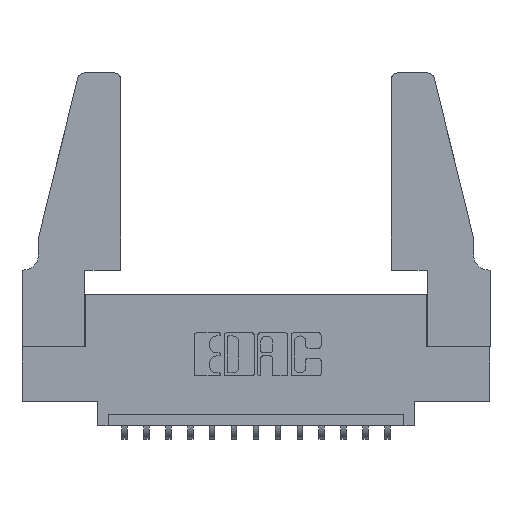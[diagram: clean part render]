
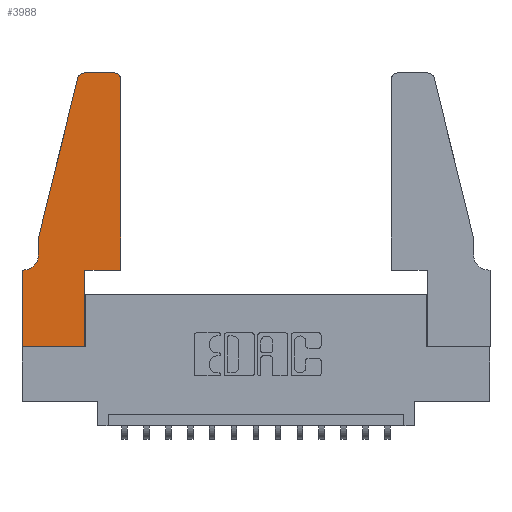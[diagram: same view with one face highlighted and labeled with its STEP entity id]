
A CAD part, top view. The second image highlights one B-rep face of the part: STEP entity #3988.
In plain terms, the highlighted planar face has unit normal (0, 0, 1).
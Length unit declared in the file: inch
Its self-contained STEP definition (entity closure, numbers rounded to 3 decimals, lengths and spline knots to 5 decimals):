
#80 = DIRECTION ( 'NONE',  ( -0.239, -0.971, 0. ) ) ;
#277 = CIRCLE ( 'NONE', #10019, 0.07 ) ;
#354 = ORIENTED_EDGE ( 'NONE', *, *, #3174, .T. ) ;
#859 = CIRCLE ( 'NONE', #9295, 0.03 ) ;
#960 = EDGE_CURVE ( 'NONE', #12987, #6282, #12792, .T. ) ;
#1003 = CARTESIAN_POINT ( 'NONE',  ( 0., 0.35, 0.37 ) ) ;
#1084 = CIRCLE ( 'NONE', #4868, 0.03 ) ;
#1091 = VECTOR ( 'NONE', #2805, 39.37008 ) ;
#1187 = CARTESIAN_POINT ( 'NONE',  ( 0.4505, 0.35, 0.37 ) ) ;
#1216 = CARTESIAN_POINT ( 'NONE',  ( 0.4505, 0.35, 0.37 ) ) ;
#1389 = VERTEX_POINT ( 'NONE', #12615 ) ;
#1526 = DIRECTION ( 'NONE',  ( 0., 0., 1. ) ) ;
#1555 = VECTOR ( 'NONE', #8301, 39.37008 ) ;
#1618 = CARTESIAN_POINT ( 'NONE',  ( 0.2605, 1.25, 0.37 ) ) ;
#1669 = ORIENTED_EDGE ( 'NONE', *, *, #2639, .T. ) ;
#1764 = DIRECTION ( 'NONE',  ( 0., 1., 0. ) ) ;
#2201 = DIRECTION ( 'NONE',  ( 1., 0., 0. ) ) ;
#2376 = CARTESIAN_POINT ( 'NONE',  ( 0.4205, 1.25, 0.37 ) ) ;
#2639 = EDGE_CURVE ( 'NONE', #14025, #1389, #1084, .T. ) ;
#2805 = DIRECTION ( 'NONE',  ( 1., 0., 0. ) ) ;
#2828 = VECTOR ( 'NONE', #1764, 39.37008 ) ;
#2954 = DIRECTION ( 'NONE',  ( -1., 0., 0. ) ) ;
#3007 = LINE ( 'NONE', #6112, #11578 ) ;
#3174 = EDGE_CURVE ( 'NONE', #15746, #14275, #10976, .T. ) ;
#3208 = EDGE_LOOP ( 'NONE', ( #7378, #1669, #3851, #354, #9193, #8293, #15738, #5438, #5423, #12351, #14378, #4450 ) ) ;
#3361 = CARTESIAN_POINT ( 'NONE',  ( 0.4505, 0.35, 0.37 ) ) ;
#3488 = EDGE_CURVE ( 'NONE', #5289, #13604, #859, .T. ) ;
#3773 = CARTESIAN_POINT ( 'NONE',  ( 0.0755, 0.35, 0.37 ) ) ;
#3851 = ORIENTED_EDGE ( 'NONE', *, *, #5903, .T. ) ;
#3988 = ADVANCED_FACE ( 'NONE', ( #13448 ), #5974, .T. ) ;
#4026 = VERTEX_POINT ( 'NONE', #4763 ) ;
#4060 = VERTEX_POINT ( 'NONE', #1003 ) ;
#4179 = EDGE_CURVE ( 'NONE', #6282, #5289, #15571, .T. ) ;
#4184 = VERTEX_POINT ( 'NONE', #11095 ) ;
#4376 = EDGE_CURVE ( 'NONE', #14275, #8787, #277, .T. ) ;
#4450 = ORIENTED_EDGE ( 'NONE', *, *, #3488, .T. ) ;
#4763 = CARTESIAN_POINT ( 'NONE',  ( 0.2865, 0., 0.37 ) ) ;
#4868 = AXIS2_PLACEMENT_3D ( 'NONE', #15170, #1526, #12731 ) ;
#4936 = DIRECTION ( 'NONE',  ( 0., 0., -1. ) ) ;
#4996 = EDGE_CURVE ( 'NONE', #4184, #4026, #15457, .T. ) ;
#5127 = CARTESIAN_POINT ( 'NONE',  ( 0.2865, 0.35, 0.37 ) ) ;
#5289 = VERTEX_POINT ( 'NONE', #7428 ) ;
#5423 = ORIENTED_EDGE ( 'NONE', *, *, #16003, .T. ) ;
#5436 = CARTESIAN_POINT ( 'NONE',  ( 0., 0., 0.37 ) ) ;
#5438 = ORIENTED_EDGE ( 'NONE', *, *, #4996, .T. ) ;
#5752 = LINE ( 'NONE', #7013, #8712 ) ;
#5903 = EDGE_CURVE ( 'NONE', #1389, #15746, #3007, .T. ) ;
#5974 = PLANE ( 'NONE',  #15796 ) ;
#6083 = DIRECTION ( 'NONE',  ( 0., 0., 1. ) ) ;
#6112 = CARTESIAN_POINT ( 'NONE',  ( 0.0755, 0.5, 0.37 ) ) ;
#6240 = DIRECTION ( 'NONE',  ( -1., 0., 0. ) ) ;
#6282 = VERTEX_POINT ( 'NONE', #1187 ) ;
#6354 = CARTESIAN_POINT ( 'NONE',  ( 0.0055, 0.42, 0.37 ) ) ;
#6578 = LINE ( 'NONE', #1618, #15516 ) ;
#6843 = CARTESIAN_POINT ( 'NONE',  ( 0.0055, 0.35, 0.37 ) ) ;
#7013 = CARTESIAN_POINT ( 'NONE',  ( 0., 0., 0.37 ) ) ;
#7027 = CARTESIAN_POINT ( 'NONE',  ( 0.0755, 0.5, 0.37 ) ) ;
#7100 = DIRECTION ( 'NONE',  ( 1., 0., 0. ) ) ;
#7253 = LINE ( 'NONE', #9204, #2828 ) ;
#7378 = ORIENTED_EDGE ( 'NONE', *, *, #9332, .T. ) ;
#7428 = CARTESIAN_POINT ( 'NONE',  ( 0.4505, 1.22, 0.37 ) ) ;
#8076 = CARTESIAN_POINT ( 'NONE',  ( 0.0755, 0.42, 0.37 ) ) ;
#8264 = DIRECTION ( 'NONE',  ( 0., 0., 1. ) ) ;
#8293 = ORIENTED_EDGE ( 'NONE', *, *, #13581, .T. ) ;
#8301 = DIRECTION ( 'NONE',  ( 1., 0., 0. ) ) ;
#8445 = CARTESIAN_POINT ( 'NONE',  ( 0., 0.35, 0.37 ) ) ;
#8712 = VECTOR ( 'NONE', #13373, 39.37008 ) ;
#8772 = CARTESIAN_POINT ( 'NONE',  ( 0.0755, 0.5, 0.37 ) ) ;
#8787 = VERTEX_POINT ( 'NONE', #6843 ) ;
#8919 = LINE ( 'NONE', #3773, #12785 ) ;
#9193 = ORIENTED_EDGE ( 'NONE', *, *, #4376, .T. ) ;
#9204 = CARTESIAN_POINT ( 'NONE',  ( 0.2865, 0.35, 0.37 ) ) ;
#9295 = AXIS2_PLACEMENT_3D ( 'NONE', #14549, #8264, #7100 ) ;
#9332 = EDGE_CURVE ( 'NONE', #13604, #14025, #6578, .T. ) ;
#9541 = DIRECTION ( 'NONE',  ( 0., -1., 0. ) ) ;
#9956 = DIRECTION ( 'NONE',  ( 0., 1., 0. ) ) ;
#10019 = AXIS2_PLACEMENT_3D ( 'NONE', #6354, #4936, #6240 ) ;
#10218 = EDGE_CURVE ( 'NONE', #4060, #4184, #5752, .T. ) ;
#10976 = LINE ( 'NONE', #7027, #11195 ) ;
#11095 = CARTESIAN_POINT ( 'NONE',  ( 0., 0., 0.37 ) ) ;
#11195 = VECTOR ( 'NONE', #9541, 39.37008 ) ;
#11578 = VECTOR ( 'NONE', #80, 39.37008 ) ;
#12306 = DIRECTION ( 'NONE',  ( -1., 0., 0. ) ) ;
#12351 = ORIENTED_EDGE ( 'NONE', *, *, #960, .T. ) ;
#12444 = CARTESIAN_POINT ( 'NONE',  ( 0.284, 1.25, 0.37 ) ) ;
#12615 = CARTESIAN_POINT ( 'NONE',  ( 0.25487, 1.22718, 0.37 ) ) ;
#12731 = DIRECTION ( 'NONE',  ( 1., 0., 0. ) ) ;
#12785 = VECTOR ( 'NONE', #12306, 39.37008 ) ;
#12792 = LINE ( 'NONE', #3361, #1555 ) ;
#12987 = VERTEX_POINT ( 'NONE', #5127 ) ;
#13373 = DIRECTION ( 'NONE',  ( 0., -1., 0. ) ) ;
#13448 = FACE_OUTER_BOUND ( 'NONE', #3208, .T. ) ;
#13581 = EDGE_CURVE ( 'NONE', #8787, #4060, #8919, .T. ) ;
#13604 = VERTEX_POINT ( 'NONE', #2376 ) ;
#14025 = VERTEX_POINT ( 'NONE', #12444 ) ;
#14275 = VERTEX_POINT ( 'NONE', #8076 ) ;
#14378 = ORIENTED_EDGE ( 'NONE', *, *, #4179, .T. ) ;
#14549 = CARTESIAN_POINT ( 'NONE',  ( 0.4205, 1.22, 0.37 ) ) ;
#14800 = VECTOR ( 'NONE', #9956, 39.37008 ) ;
#15170 = CARTESIAN_POINT ( 'NONE',  ( 0.284, 1.22, 0.37 ) ) ;
#15457 = LINE ( 'NONE', #5436, #1091 ) ;
#15516 = VECTOR ( 'NONE', #2954, 39.37008 ) ;
#15571 = LINE ( 'NONE', #1216, #14800 ) ;
#15738 = ORIENTED_EDGE ( 'NONE', *, *, #10218, .T. ) ;
#15746 = VERTEX_POINT ( 'NONE', #8772 ) ;
#15796 = AXIS2_PLACEMENT_3D ( 'NONE', #8445, #6083, #2201 ) ;
#16003 = EDGE_CURVE ( 'NONE', #4026, #12987, #7253, .T. ) ;
